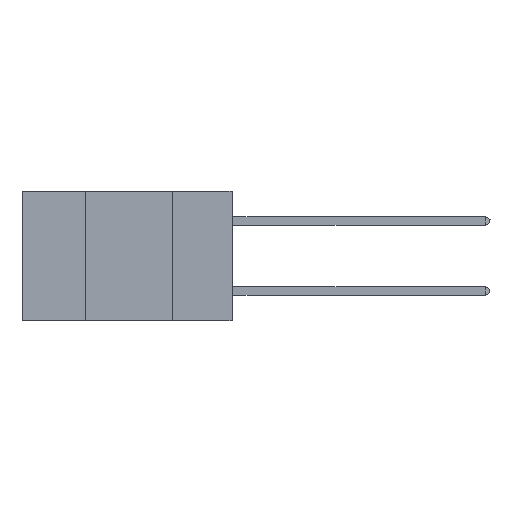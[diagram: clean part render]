
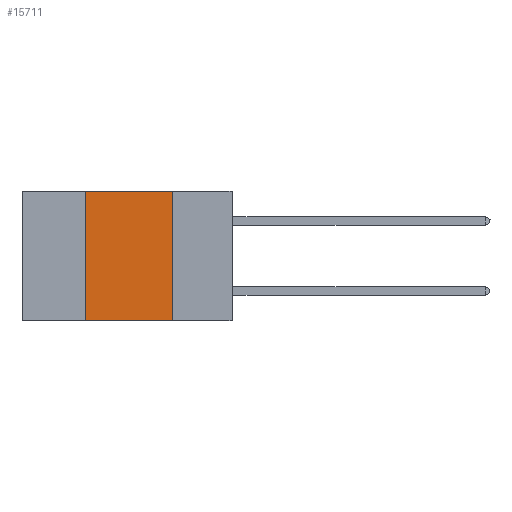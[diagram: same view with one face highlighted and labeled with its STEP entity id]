
A CAD part, left-side view. The second image highlights one B-rep face of the part: STEP entity #15711.
In plain terms, the highlighted planar face has unit normal (-1, 0, 0).
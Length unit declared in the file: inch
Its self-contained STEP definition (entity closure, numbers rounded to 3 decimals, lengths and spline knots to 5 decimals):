
#142 = ORIENTED_EDGE ( 'NONE', *, *, #14630, .F. ) ;
#453 = CARTESIAN_POINT ( 'NONE',  ( 0., 0.6, 0. ) ) ;
#831 = EDGE_CURVE ( 'NONE', #11238, #3946, #5861, .T. ) ;
#1149 = AXIS2_PLACEMENT_3D ( 'NONE', #453, #3246, #13308 ) ;
#1566 = LINE ( 'NONE', #2766, #3856 ) ;
#2766 = CARTESIAN_POINT ( 'NONE',  ( 0., 0.17, 0. ) ) ;
#3178 = CARTESIAN_POINT ( 'NONE',  ( 0., 0.42, 0. ) ) ;
#3246 = DIRECTION ( 'NONE',  ( 1., 0., 0. ) ) ;
#3266 = LINE ( 'NONE', #3178, #11315 ) ;
#3856 = VECTOR ( 'NONE', #5745, 39.37008 ) ;
#3946 = VERTEX_POINT ( 'NONE', #5121 ) ;
#4263 = DIRECTION ( 'NONE',  ( 0., -1., 0. ) ) ;
#5121 = CARTESIAN_POINT ( 'NONE',  ( 0., 0.17, 0. ) ) ;
#5745 = DIRECTION ( 'NONE',  ( 0., 0., -1. ) ) ;
#5861 = LINE ( 'NONE', #9971, #10927 ) ;
#5871 = DIRECTION ( 'NONE',  ( 0., 0., 1. ) ) ;
#6464 = CARTESIAN_POINT ( 'NONE',  ( 0., 0.42, 0. ) ) ;
#7259 = VECTOR ( 'NONE', #4263, 39.37008 ) ;
#8064 = ORIENTED_EDGE ( 'NONE', *, *, #831, .F. ) ;
#8134 = VERTEX_POINT ( 'NONE', #10285 ) ;
#8752 = DIRECTION ( 'NONE',  ( 0., -1., 0. ) ) ;
#8806 = EDGE_CURVE ( 'NONE', #14065, #8134, #17105, .T. ) ;
#9372 = EDGE_LOOP ( 'NONE', ( #13714, #8064, #142, #15191 ) ) ;
#9971 = CARTESIAN_POINT ( 'NONE',  ( 0., 0.6, 0. ) ) ;
#10285 = CARTESIAN_POINT ( 'NONE',  ( 0., 0.17, -0.37 ) ) ;
#10927 = VECTOR ( 'NONE', #8752, 39.37008 ) ;
#11238 = VERTEX_POINT ( 'NONE', #6464 ) ;
#11315 = VECTOR ( 'NONE', #5871, 39.37008 ) ;
#11542 = PLANE ( 'NONE',  #1149 ) ;
#13308 = DIRECTION ( 'NONE',  ( 0., 0., -1. ) ) ;
#13714 = ORIENTED_EDGE ( 'NONE', *, *, #14134, .F. ) ;
#14065 = VERTEX_POINT ( 'NONE', #14325 ) ;
#14134 = EDGE_CURVE ( 'NONE', #3946, #8134, #1566, .T. ) ;
#14325 = CARTESIAN_POINT ( 'NONE',  ( 0., 0.42, -0.37 ) ) ;
#14609 = FACE_OUTER_BOUND ( 'NONE', #9372, .T. ) ;
#14630 = EDGE_CURVE ( 'NONE', #14065, #11238, #3266, .T. ) ;
#15191 = ORIENTED_EDGE ( 'NONE', *, *, #8806, .T. ) ;
#15711 = ADVANCED_FACE ( 'NONE', ( #14609 ), #11542, .F. ) ;
#17105 = LINE ( 'NONE', #18236, #7259 ) ;
#18236 = CARTESIAN_POINT ( 'NONE',  ( 0., 0.6, -0.37 ) ) ;
